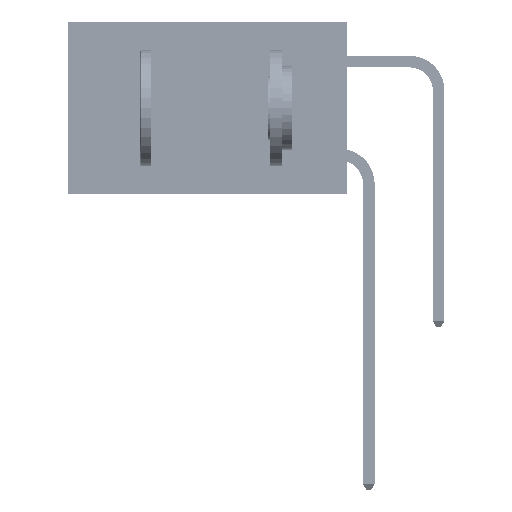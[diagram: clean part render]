
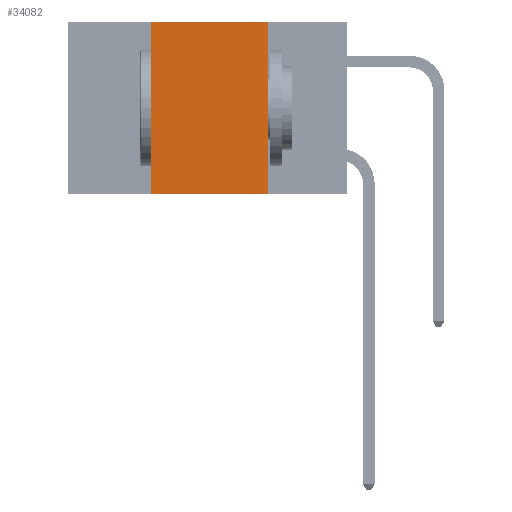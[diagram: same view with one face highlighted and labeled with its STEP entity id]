
A CAD part, left-side view. The second image highlights one B-rep face of the part: STEP entity #34082.
In plain terms, the highlighted planar face has unit normal (-1, 0, 0).
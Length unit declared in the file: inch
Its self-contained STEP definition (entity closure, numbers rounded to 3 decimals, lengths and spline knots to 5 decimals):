
#205 = CARTESIAN_POINT ( 'NONE',  ( 0., 0.42, -0.37 ) ) ;
#1050 = AXIS2_PLACEMENT_3D ( 'NONE', #11014, #37359, #14832 ) ;
#1249 = EDGE_CURVE ( 'NONE', #34930, #3467, #6423, .T. ) ;
#1993 = VECTOR ( 'NONE', #18893, 39.37008 ) ;
#2997 = VECTOR ( 'NONE', #16991, 39.37008 ) ;
#3143 = EDGE_LOOP ( 'NONE', ( #25612, #47971, #39162, #3584 ) ) ;
#3467 = VERTEX_POINT ( 'NONE', #10138 ) ;
#3584 = ORIENTED_EDGE ( 'NONE', *, *, #1249, .T. ) ;
#3837 = DIRECTION ( 'NONE',  ( 0., -1., 0. ) ) ;
#6423 = LINE ( 'NONE', #30446, #36576 ) ;
#10138 = CARTESIAN_POINT ( 'NONE',  ( 0., 0.17, -0.37 ) ) ;
#11014 = CARTESIAN_POINT ( 'NONE',  ( 0., 0.6, 0. ) ) ;
#12304 = LINE ( 'NONE', #37603, #1993 ) ;
#14832 = DIRECTION ( 'NONE',  ( 0., 0., -1. ) ) ;
#16734 = EDGE_CURVE ( 'NONE', #34930, #17874, #12304, .T. ) ;
#16991 = DIRECTION ( 'NONE',  ( 0., 0., -1. ) ) ;
#17874 = VERTEX_POINT ( 'NONE', #31653 ) ;
#18363 = VERTEX_POINT ( 'NONE', #41994 ) ;
#18893 = DIRECTION ( 'NONE',  ( 0., 0., 1. ) ) ;
#22249 = VECTOR ( 'NONE', #40687, 39.37008 ) ;
#25612 = ORIENTED_EDGE ( 'NONE', *, *, #36888, .F. ) ;
#30446 = CARTESIAN_POINT ( 'NONE',  ( 0., 0.6, -0.37 ) ) ;
#31653 = CARTESIAN_POINT ( 'NONE',  ( 0., 0.42, 0. ) ) ;
#33555 = PLANE ( 'NONE',  #1050 ) ;
#34082 = ADVANCED_FACE ( 'NONE', ( #48572 ), #33555, .F. ) ;
#34930 = VERTEX_POINT ( 'NONE', #205 ) ;
#36576 = VECTOR ( 'NONE', #3837, 39.37008 ) ;
#36878 = CARTESIAN_POINT ( 'NONE',  ( 0., 0.6, 0. ) ) ;
#36888 = EDGE_CURVE ( 'NONE', #18363, #3467, #40977, .T. ) ;
#37359 = DIRECTION ( 'NONE',  ( 1., 0., 0. ) ) ;
#37603 = CARTESIAN_POINT ( 'NONE',  ( 0., 0.42, 0. ) ) ;
#39162 = ORIENTED_EDGE ( 'NONE', *, *, #16734, .F. ) ;
#40687 = DIRECTION ( 'NONE',  ( 0., -1., 0. ) ) ;
#40977 = LINE ( 'NONE', #43311, #2997 ) ;
#41994 = CARTESIAN_POINT ( 'NONE',  ( 0., 0.17, 0. ) ) ;
#42242 = LINE ( 'NONE', #36878, #22249 ) ;
#42303 = EDGE_CURVE ( 'NONE', #17874, #18363, #42242, .T. ) ;
#43311 = CARTESIAN_POINT ( 'NONE',  ( 0., 0.17, 0. ) ) ;
#47971 = ORIENTED_EDGE ( 'NONE', *, *, #42303, .F. ) ;
#48572 = FACE_OUTER_BOUND ( 'NONE', #3143, .T. ) ;
